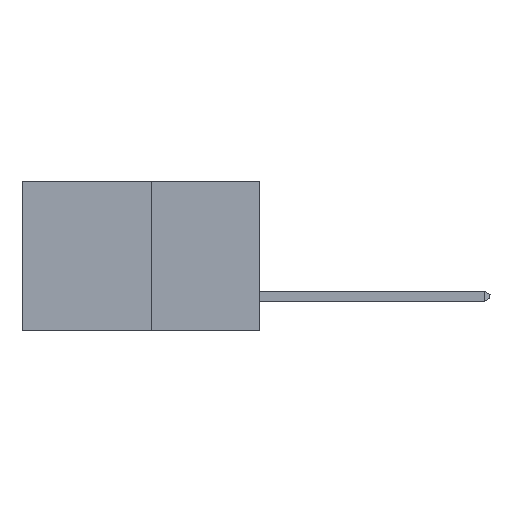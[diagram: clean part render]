
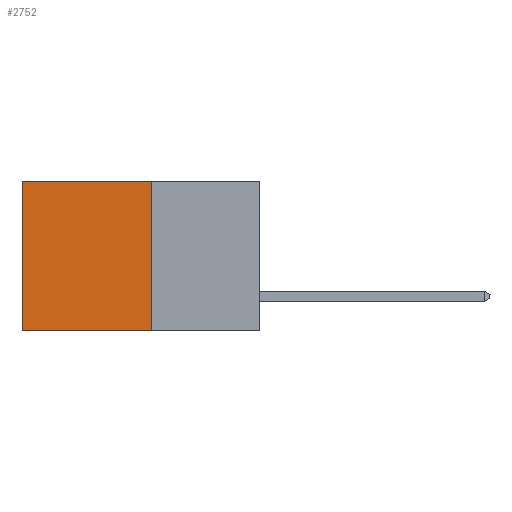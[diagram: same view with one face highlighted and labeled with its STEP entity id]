
A CAD part, left-side view. The second image highlights one B-rep face of the part: STEP entity #2752.
In plain terms, the highlighted planar face has unit normal (-1, 0, 0).
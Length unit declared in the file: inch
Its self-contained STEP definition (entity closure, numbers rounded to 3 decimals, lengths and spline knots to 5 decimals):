
#7 = ORIENTED_EDGE ( 'NONE', *, *, #8793, .F. ) ;
#26 = EDGE_LOOP ( 'NONE', ( #5817, #7, #600, #5330 ) ) ;
#600 = ORIENTED_EDGE ( 'NONE', *, *, #2608, .F. ) ;
#766 = CARTESIAN_POINT ( 'NONE',  ( 0.277, 0.59, -0.37 ) ) ;
#1042 = VERTEX_POINT ( 'NONE', #2760 ) ;
#1477 = LINE ( 'NONE', #4423, #6528 ) ;
#1556 = VECTOR ( 'NONE', #5366, 39.37008 ) ;
#1592 = EDGE_CURVE ( 'NONE', #5216, #4201, #1477, .T. ) ;
#1904 = VECTOR ( 'NONE', #5276, 39.37008 ) ;
#2608 = EDGE_CURVE ( 'NONE', #5216, #7453, #3455, .T. ) ;
#2701 = LINE ( 'NONE', #766, #8116 ) ;
#2752 = ADVANCED_FACE ( 'NONE', ( #3298 ), #3082, .F. ) ;
#2760 = CARTESIAN_POINT ( 'NONE',  ( 0.277, 0.59, -0.37 ) ) ;
#3047 = DIRECTION ( 'NONE',  ( 1., 0., 0. ) ) ;
#3067 = AXIS2_PLACEMENT_3D ( 'NONE', #5031, #3047, #7485 ) ;
#3082 = PLANE ( 'NONE',  #3067 ) ;
#3298 = FACE_OUTER_BOUND ( 'NONE', #26, .T. ) ;
#3455 = LINE ( 'NONE', #7189, #1556 ) ;
#3819 = LINE ( 'NONE', #8060, #1904 ) ;
#4201 = VERTEX_POINT ( 'NONE', #7677 ) ;
#4423 = CARTESIAN_POINT ( 'NONE',  ( 0.277, 0.27, 0. ) ) ;
#5031 = CARTESIAN_POINT ( 'NONE',  ( 0.277, 0.27, -0.37 ) ) ;
#5216 = VERTEX_POINT ( 'NONE', #8782 ) ;
#5276 = DIRECTION ( 'NONE',  ( 0., 1., 0. ) ) ;
#5330 = ORIENTED_EDGE ( 'NONE', *, *, #1592, .T. ) ;
#5366 = DIRECTION ( 'NONE',  ( 0., 0., -1. ) ) ;
#5803 = DIRECTION ( 'NONE',  ( 0., 0., -1. ) ) ;
#5817 = ORIENTED_EDGE ( 'NONE', *, *, #7963, .T. ) ;
#6333 = DIRECTION ( 'NONE',  ( 0., 1., 0. ) ) ;
#6528 = VECTOR ( 'NONE', #6333, 39.37008 ) ;
#7189 = CARTESIAN_POINT ( 'NONE',  ( 0.277, 0.27, -0.37 ) ) ;
#7453 = VERTEX_POINT ( 'NONE', #8556 ) ;
#7485 = DIRECTION ( 'NONE',  ( 0., 0., -1. ) ) ;
#7677 = CARTESIAN_POINT ( 'NONE',  ( 0.277, 0.59, 0. ) ) ;
#7963 = EDGE_CURVE ( 'NONE', #4201, #1042, #2701, .T. ) ;
#8060 = CARTESIAN_POINT ( 'NONE',  ( 0.277, 0.27, -0.37 ) ) ;
#8116 = VECTOR ( 'NONE', #5803, 39.37008 ) ;
#8556 = CARTESIAN_POINT ( 'NONE',  ( 0.277, 0.27, -0.37 ) ) ;
#8782 = CARTESIAN_POINT ( 'NONE',  ( 0.277, 0.27, 0. ) ) ;
#8793 = EDGE_CURVE ( 'NONE', #7453, #1042, #3819, .T. ) ;
